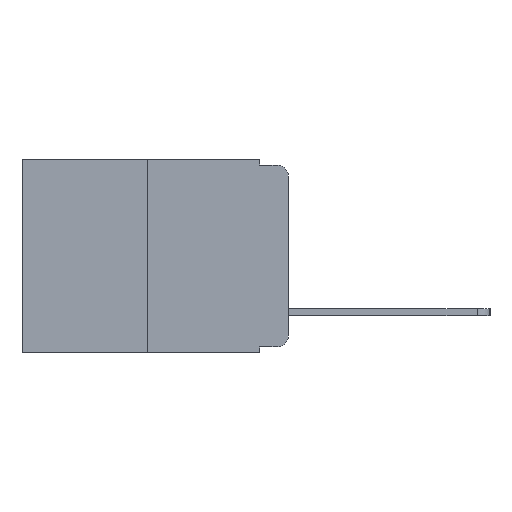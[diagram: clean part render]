
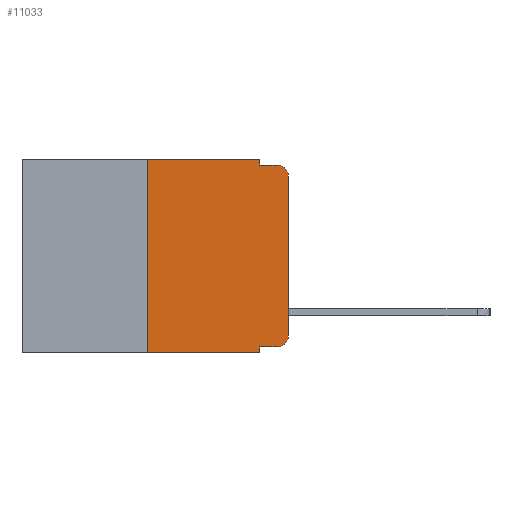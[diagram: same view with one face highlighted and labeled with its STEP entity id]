
A CAD part, left-side view. The second image highlights one B-rep face of the part: STEP entity #11033.
In plain terms, the highlighted planar face has unit normal (-1, 0, 0).
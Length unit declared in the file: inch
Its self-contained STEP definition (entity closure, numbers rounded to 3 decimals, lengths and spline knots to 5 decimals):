
#175 = EDGE_CURVE ( 'NONE', #13973, #7853, #7016, .T. ) ;
#772 = DIRECTION ( 'NONE',  ( 0., 0., 1. ) ) ;
#812 = CARTESIAN_POINT ( 'NONE',  ( 0., 0.473, 0. ) ) ;
#1163 = LINE ( 'NONE', #17208, #4901 ) ;
#1332 = ORIENTED_EDGE ( 'NONE', *, *, #16549, .T. ) ;
#1750 = EDGE_LOOP ( 'NONE', ( #11359, #16755, #21336, #7668, #13080, #4511, #14199, #5071, #20005, #1332 ) ) ;
#2636 = EDGE_CURVE ( 'NONE', #13143, #7853, #17858, .T. ) ;
#2649 = CARTESIAN_POINT ( 'NONE',  ( 0., 0.25, 0. ) ) ;
#2658 = DIRECTION ( 'NONE',  ( 0., 0., -1. ) ) ;
#2692 = VECTOR ( 'NONE', #6141, 39.37008 ) ;
#3669 = VERTEX_POINT ( 'NONE', #16879 ) ;
#3814 = CARTESIAN_POINT ( 'NONE',  ( 0., 0.02, -0.313 ) ) ;
#4511 = ORIENTED_EDGE ( 'NONE', *, *, #21177, .F. ) ;
#4636 = VERTEX_POINT ( 'NONE', #21471 ) ;
#4744 = DIRECTION ( 'NONE',  ( 0., -1., 0. ) ) ;
#4901 = VECTOR ( 'NONE', #22465, 39.37008 ) ;
#4961 = CARTESIAN_POINT ( 'NONE',  ( 0., 0.051, -0.01 ) ) ;
#5071 = ORIENTED_EDGE ( 'NONE', *, *, #18885, .F. ) ;
#5095 = EDGE_CURVE ( 'NONE', #7504, #13143, #22589, .T. ) ;
#5231 = LINE ( 'NONE', #12480, #18553 ) ;
#5662 = DIRECTION ( 'NONE',  ( 0., 0., -1. ) ) ;
#5762 = CARTESIAN_POINT ( 'NONE',  ( 0., 0.25, 0. ) ) ;
#6103 = DIRECTION ( 'NONE',  ( 0., -1., 0. ) ) ;
#6141 = DIRECTION ( 'NONE',  ( 0., -1., 0. ) ) ;
#6560 = CARTESIAN_POINT ( 'NONE',  ( 0., 0.473, -0.343 ) ) ;
#6561 = CARTESIAN_POINT ( 'NONE',  ( 0., 0.02, -0.03 ) ) ;
#6691 = AXIS2_PLACEMENT_3D ( 'NONE', #6561, #7959, #8358 ) ;
#6865 = CARTESIAN_POINT ( 'NONE',  ( 0., 0.051, 0. ) ) ;
#7016 = LINE ( 'NONE', #10925, #2692 ) ;
#7504 = VERTEX_POINT ( 'NONE', #21474 ) ;
#7668 = ORIENTED_EDGE ( 'NONE', *, *, #22338, .F. ) ;
#7853 = VERTEX_POINT ( 'NONE', #14767 ) ;
#7959 = DIRECTION ( 'NONE',  ( -1., 0., 0. ) ) ;
#8049 = FACE_OUTER_BOUND ( 'NONE', #1750, .T. ) ;
#8358 = DIRECTION ( 'NONE',  ( 0., 0., -1. ) ) ;
#8611 = VECTOR ( 'NONE', #14380, 39.37008 ) ;
#8782 = EDGE_CURVE ( 'NONE', #11452, #20203, #5231, .T. ) ;
#9361 = AXIS2_PLACEMENT_3D ( 'NONE', #3814, #16587, #5662 ) ;
#9691 = VERTEX_POINT ( 'NONE', #14097 ) ;
#10925 = CARTESIAN_POINT ( 'NONE',  ( 0., 0.051, -0.01 ) ) ;
#11033 = ADVANCED_FACE ( 'NONE', ( #8049 ), #11785, .F. ) ;
#11359 = ORIENTED_EDGE ( 'NONE', *, *, #5095, .T. ) ;
#11452 = VERTEX_POINT ( 'NONE', #5762 ) ;
#11785 = PLANE ( 'NONE',  #15646 ) ;
#12480 = CARTESIAN_POINT ( 'NONE',  ( 0., 0.473, 0. ) ) ;
#12726 = CARTESIAN_POINT ( 'NONE',  ( 0., 0.02, -0.333 ) ) ;
#13061 = DIRECTION ( 'NONE',  ( 0., 0., -1. ) ) ;
#13080 = ORIENTED_EDGE ( 'NONE', *, *, #8782, .F. ) ;
#13143 = VERTEX_POINT ( 'NONE', #15370 ) ;
#13220 = VECTOR ( 'NONE', #17307, 39.37008 ) ;
#13472 = LINE ( 'NONE', #16121, #8611 ) ;
#13624 = DIRECTION ( 'NONE',  ( 1., 0., 0. ) ) ;
#13959 = VECTOR ( 'NONE', #13061, 39.37008 ) ;
#13973 = VERTEX_POINT ( 'NONE', #4961 ) ;
#14097 = CARTESIAN_POINT ( 'NONE',  ( 0., 0.25, -0.343 ) ) ;
#14199 = ORIENTED_EDGE ( 'NONE', *, *, #19172, .T. ) ;
#14380 = DIRECTION ( 'NONE',  ( 0., -1., 0. ) ) ;
#14767 = CARTESIAN_POINT ( 'NONE',  ( 0., 0.02, -0.01 ) ) ;
#15370 = CARTESIAN_POINT ( 'NONE',  ( 0., 0., -0.03 ) ) ;
#15646 = AXIS2_PLACEMENT_3D ( 'NONE', #812, #13624, #2658 ) ;
#16121 = CARTESIAN_POINT ( 'NONE',  ( 0., 0.051, -0.333 ) ) ;
#16216 = LINE ( 'NONE', #18376, #13959 ) ;
#16549 = EDGE_CURVE ( 'NONE', #19431, #7504, #16645, .T. ) ;
#16587 = DIRECTION ( 'NONE',  ( -1., 0., 0. ) ) ;
#16645 = CIRCLE ( 'NONE', #9361, 0.02 ) ;
#16755 = ORIENTED_EDGE ( 'NONE', *, *, #2636, .T. ) ;
#16879 = CARTESIAN_POINT ( 'NONE',  ( 0., 0.051, -0.343 ) ) ;
#17208 = CARTESIAN_POINT ( 'NONE',  ( 0., 0.051, 0. ) ) ;
#17307 = DIRECTION ( 'NONE',  ( 0., 0., 1. ) ) ;
#17335 = LINE ( 'NONE', #6560, #21357 ) ;
#17721 = EDGE_CURVE ( 'NONE', #4636, #19431, #13472, .T. ) ;
#17858 = CIRCLE ( 'NONE', #6691, 0.02 ) ;
#18376 = CARTESIAN_POINT ( 'NONE',  ( 0., 0.051, 0. ) ) ;
#18553 = VECTOR ( 'NONE', #6103, 39.37008 ) ;
#18885 = EDGE_CURVE ( 'NONE', #4636, #3669, #16216, .T. ) ;
#19172 = EDGE_CURVE ( 'NONE', #9691, #3669, #17335, .T. ) ;
#19431 = VERTEX_POINT ( 'NONE', #12726 ) ;
#20005 = ORIENTED_EDGE ( 'NONE', *, *, #17721, .T. ) ;
#20203 = VERTEX_POINT ( 'NONE', #6865 ) ;
#20972 = CARTESIAN_POINT ( 'NONE',  ( 0., 0., 0. ) ) ;
#21177 = EDGE_CURVE ( 'NONE', #9691, #11452, #22564, .T. ) ;
#21336 = ORIENTED_EDGE ( 'NONE', *, *, #175, .F. ) ;
#21357 = VECTOR ( 'NONE', #4744, 39.37008 ) ;
#21471 = CARTESIAN_POINT ( 'NONE',  ( 0., 0.051, -0.333 ) ) ;
#21474 = CARTESIAN_POINT ( 'NONE',  ( 0., 0., -0.313 ) ) ;
#22043 = VECTOR ( 'NONE', #772, 39.37008 ) ;
#22338 = EDGE_CURVE ( 'NONE', #20203, #13973, #1163, .T. ) ;
#22465 = DIRECTION ( 'NONE',  ( 0., 0., -1. ) ) ;
#22564 = LINE ( 'NONE', #2649, #13220 ) ;
#22589 = LINE ( 'NONE', #20972, #22043 ) ;
